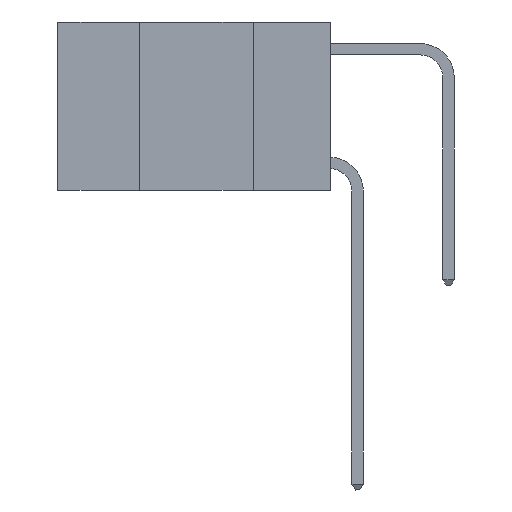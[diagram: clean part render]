
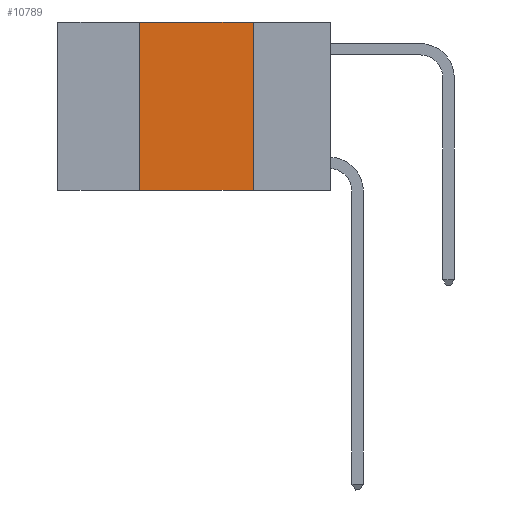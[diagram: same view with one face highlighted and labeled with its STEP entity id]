
A CAD part, left-side view. The second image highlights one B-rep face of the part: STEP entity #10789.
In plain terms, the highlighted planar face has unit normal (-1, 0, 0).
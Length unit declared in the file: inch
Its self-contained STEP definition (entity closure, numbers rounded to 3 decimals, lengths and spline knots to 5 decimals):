
#359 = FACE_OUTER_BOUND ( 'NONE', #10454, .T. ) ;
#506 = CARTESIAN_POINT ( 'NONE',  ( 0., 0.17, 0. ) ) ;
#581 = DIRECTION ( 'NONE',  ( 0., 0., -1. ) ) ;
#1485 = CARTESIAN_POINT ( 'NONE',  ( 0., 0.42, -0.37 ) ) ;
#2278 = LINE ( 'NONE', #506, #10149 ) ;
#2470 = EDGE_CURVE ( 'NONE', #12992, #6344, #12904, .T. ) ;
#2805 = DIRECTION ( 'NONE',  ( 0., 0., -1. ) ) ;
#3005 = CARTESIAN_POINT ( 'NONE',  ( 0., 0.42, 0. ) ) ;
#3889 = CARTESIAN_POINT ( 'NONE',  ( 0., 0.42, 0. ) ) ;
#4315 = EDGE_CURVE ( 'NONE', #6344, #6085, #2278, .T. ) ;
#4333 = EDGE_CURVE ( 'NONE', #13246, #12992, #12381, .T. ) ;
#4378 = EDGE_CURVE ( 'NONE', #13246, #6085, #6855, .T. ) ;
#5014 = VECTOR ( 'NONE', #6490, 39.37008 ) ;
#5461 = CARTESIAN_POINT ( 'NONE',  ( 0., 0.6, 0. ) ) ;
#5946 = PLANE ( 'NONE',  #8017 ) ;
#6085 = VERTEX_POINT ( 'NONE', #12512 ) ;
#6344 = VERTEX_POINT ( 'NONE', #12806 ) ;
#6490 = DIRECTION ( 'NONE',  ( 0., -1., 0. ) ) ;
#6855 = LINE ( 'NONE', #10978, #11779 ) ;
#6944 = DIRECTION ( 'NONE',  ( 1., 0., 0. ) ) ;
#7053 = DIRECTION ( 'NONE',  ( 0., -1., 0. ) ) ;
#8017 = AXIS2_PLACEMENT_3D ( 'NONE', #12829, #6944, #581 ) ;
#8989 = DIRECTION ( 'NONE',  ( 0., 0., 1. ) ) ;
#9835 = VECTOR ( 'NONE', #8989, 39.37008 ) ;
#10149 = VECTOR ( 'NONE', #2805, 39.37008 ) ;
#10412 = ORIENTED_EDGE ( 'NONE', *, *, #4315, .F. ) ;
#10454 = EDGE_LOOP ( 'NONE', ( #10412, #10481, #10572, #10587 ) ) ;
#10481 = ORIENTED_EDGE ( 'NONE', *, *, #2470, .F. ) ;
#10572 = ORIENTED_EDGE ( 'NONE', *, *, #4333, .F. ) ;
#10587 = ORIENTED_EDGE ( 'NONE', *, *, #4378, .T. ) ;
#10789 = ADVANCED_FACE ( 'NONE', ( #359 ), #5946, .F. ) ;
#10978 = CARTESIAN_POINT ( 'NONE',  ( 0., 0.6, -0.37 ) ) ;
#11779 = VECTOR ( 'NONE', #7053, 39.37008 ) ;
#12381 = LINE ( 'NONE', #3889, #9835 ) ;
#12512 = CARTESIAN_POINT ( 'NONE',  ( 0., 0.17, -0.37 ) ) ;
#12806 = CARTESIAN_POINT ( 'NONE',  ( 0., 0.17, 0. ) ) ;
#12829 = CARTESIAN_POINT ( 'NONE',  ( 0., 0.6, 0. ) ) ;
#12904 = LINE ( 'NONE', #5461, #5014 ) ;
#12992 = VERTEX_POINT ( 'NONE', #3005 ) ;
#13246 = VERTEX_POINT ( 'NONE', #1485 ) ;
